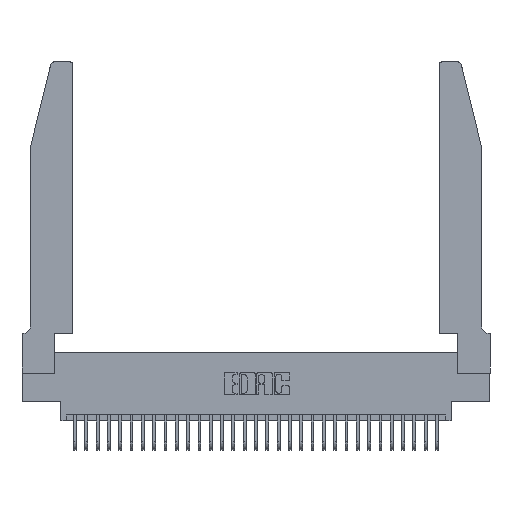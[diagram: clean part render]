
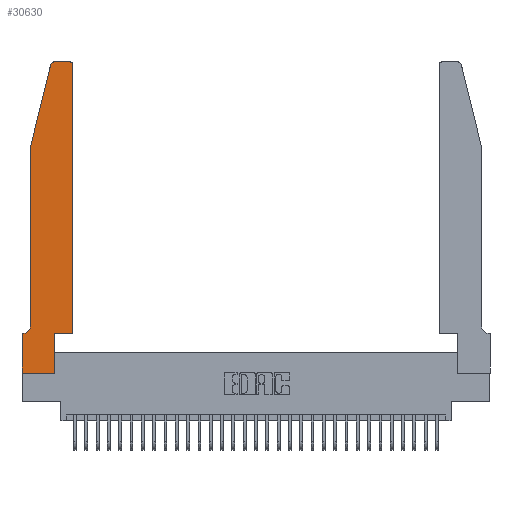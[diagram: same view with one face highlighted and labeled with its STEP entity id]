
A CAD part, top view. The second image highlights one B-rep face of the part: STEP entity #30630.
In plain terms, the highlighted planar face has unit normal (0, 0, 1).
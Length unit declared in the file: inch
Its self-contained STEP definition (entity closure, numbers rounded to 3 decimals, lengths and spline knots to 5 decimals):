
#262 = VECTOR ( 'NONE', #32092, 39.37008 ) ;
#339 = ORIENTED_EDGE ( 'NONE', *, *, #18833, .T. ) ;
#439 = CARTESIAN_POINT ( 'NONE',  ( 0.4205, 2.75, 0.37 ) ) ;
#1044 = EDGE_CURVE ( 'NONE', #23796, #20336, #15016, .T. ) ;
#1236 = EDGE_CURVE ( 'NONE', #20336, #14834, #1982, .T. ) ;
#1245 = VECTOR ( 'NONE', #25165, 39.37008 ) ;
#1545 = CARTESIAN_POINT ( 'NONE',  ( 0.25487, 2.72718, 0.37 ) ) ;
#1982 = CIRCLE ( 'NONE', #18334, 0.07 ) ;
#2623 = EDGE_LOOP ( 'NONE', ( #7126, #8928, #11662, #19348, #32763, #8503, #13892, #15949, #14632, #13035, #339, #10388 ) ) ;
#2801 = CARTESIAN_POINT ( 'NONE',  ( 0.0755, 2., 0.37 ) ) ;
#4645 = DIRECTION ( 'NONE',  ( 0., 1., 0. ) ) ;
#4680 = DIRECTION ( 'NONE',  ( 0., 0., -1. ) ) ;
#4824 = LINE ( 'NONE', #33565, #27201 ) ;
#4908 = DIRECTION ( 'NONE',  ( -1., 0., 0. ) ) ;
#6278 = VERTEX_POINT ( 'NONE', #18532 ) ;
#6332 = CARTESIAN_POINT ( 'NONE',  ( 0.284, 2.72, 0.37 ) ) ;
#6492 = DIRECTION ( 'NONE',  ( 1., 0., 0. ) ) ;
#7126 = ORIENTED_EDGE ( 'NONE', *, *, #12984, .T. ) ;
#7572 = VERTEX_POINT ( 'NONE', #22882 ) ;
#8291 = CARTESIAN_POINT ( 'NONE',  ( 0.0755, 2., 0.37 ) ) ;
#8503 = ORIENTED_EDGE ( 'NONE', *, *, #16036, .T. ) ;
#8522 = PLANE ( 'NONE',  #24957 ) ;
#8745 = DIRECTION ( 'NONE',  ( 1., 0., 0. ) ) ;
#8775 = CARTESIAN_POINT ( 'NONE',  ( 0.0055, 0.35, 0.37 ) ) ;
#8928 = ORIENTED_EDGE ( 'NONE', *, *, #31113, .T. ) ;
#9023 = CARTESIAN_POINT ( 'NONE',  ( 0.4505, 0.35, 0.37 ) ) ;
#9468 = DIRECTION ( 'NONE',  ( 0., -1., 0. ) ) ;
#9944 = VERTEX_POINT ( 'NONE', #31047 ) ;
#9985 = LINE ( 'NONE', #21358, #29141 ) ;
#10060 = EDGE_CURVE ( 'NONE', #6278, #31861, #24476, .T. ) ;
#10287 = DIRECTION ( 'NONE',  ( 1., 0., 0. ) ) ;
#10388 = ORIENTED_EDGE ( 'NONE', *, *, #11906, .T. ) ;
#11662 = ORIENTED_EDGE ( 'NONE', *, *, #32304, .T. ) ;
#11906 = EDGE_CURVE ( 'NONE', #7572, #33193, #21946, .T. ) ;
#12168 = EDGE_CURVE ( 'NONE', #9944, #29041, #4824, .T. ) ;
#12381 = FACE_OUTER_BOUND ( 'NONE', #2623, .T. ) ;
#12514 = AXIS2_PLACEMENT_3D ( 'NONE', #6332, #27166, #24223 ) ;
#12544 = CARTESIAN_POINT ( 'NONE',  ( 0., 0., 0.37 ) ) ;
#12796 = LINE ( 'NONE', #9023, #26636 ) ;
#12984 = EDGE_CURVE ( 'NONE', #33193, #17406, #9985, .T. ) ;
#13035 = ORIENTED_EDGE ( 'NONE', *, *, #16805, .T. ) ;
#13427 = VECTOR ( 'NONE', #18151, 39.37008 ) ;
#13646 = CARTESIAN_POINT ( 'NONE',  ( 0., 0., 0.37 ) ) ;
#13892 = ORIENTED_EDGE ( 'NONE', *, *, #10060, .T. ) ;
#14632 = ORIENTED_EDGE ( 'NONE', *, *, #12168, .T. ) ;
#14834 = VERTEX_POINT ( 'NONE', #8775 ) ;
#15016 = LINE ( 'NONE', #19865, #18705 ) ;
#15091 = VECTOR ( 'NONE', #10287, 39.37008 ) ;
#15474 = DIRECTION ( 'NONE',  ( 0., 1., 0. ) ) ;
#15493 = CARTESIAN_POINT ( 'NONE',  ( 0., 0., 0.37 ) ) ;
#15949 = ORIENTED_EDGE ( 'NONE', *, *, #26826, .T. ) ;
#16036 = EDGE_CURVE ( 'NONE', #14834, #6278, #31419, .T. ) ;
#16187 = CARTESIAN_POINT ( 'NONE',  ( 0., 0.35, 0.37 ) ) ;
#16805 = EDGE_CURVE ( 'NONE', #29041, #26132, #22052, .T. ) ;
#17406 = VERTEX_POINT ( 'NONE', #31102 ) ;
#17698 = CARTESIAN_POINT ( 'NONE',  ( 0.0755, 0.35, 0.37 ) ) ;
#18013 = CARTESIAN_POINT ( 'NONE',  ( 0.0755, 0.42, 0.37 ) ) ;
#18151 = DIRECTION ( 'NONE',  ( 1., 0., 0. ) ) ;
#18262 = DIRECTION ( 'NONE',  ( -1., 0., 0. ) ) ;
#18334 = AXIS2_PLACEMENT_3D ( 'NONE', #33453, #4680, #4908 ) ;
#18532 = CARTESIAN_POINT ( 'NONE',  ( 0., 0.35, 0.37 ) ) ;
#18705 = VECTOR ( 'NONE', #9468, 39.37008 ) ;
#18833 = EDGE_CURVE ( 'NONE', #26132, #7572, #12796, .T. ) ;
#19348 = ORIENTED_EDGE ( 'NONE', *, *, #1044, .T. ) ;
#19865 = CARTESIAN_POINT ( 'NONE',  ( 0.0755, 2., 0.37 ) ) ;
#20336 = VERTEX_POINT ( 'NONE', #18013 ) ;
#20381 = LINE ( 'NONE', #15493, #13427 ) ;
#21134 = DIRECTION ( 'NONE',  ( 0., 0., 1. ) ) ;
#21358 = CARTESIAN_POINT ( 'NONE',  ( 0.2605, 2.75, 0.37 ) ) ;
#21448 = DIRECTION ( 'NONE',  ( 0., 0., 1. ) ) ;
#21946 = CIRCLE ( 'NONE', #28947, 0.03 ) ;
#22052 = LINE ( 'NONE', #23327, #15091 ) ;
#22882 = CARTESIAN_POINT ( 'NONE',  ( 0.4505, 2.72, 0.37 ) ) ;
#23327 = CARTESIAN_POINT ( 'NONE',  ( 0.4505, 0.35, 0.37 ) ) ;
#23633 = CARTESIAN_POINT ( 'NONE',  ( 0.4205, 2.72, 0.37 ) ) ;
#23725 = VECTOR ( 'NONE', #18262, 39.37008 ) ;
#23796 = VERTEX_POINT ( 'NONE', #2801 ) ;
#24223 = DIRECTION ( 'NONE',  ( 1., 0., 0. ) ) ;
#24297 = DIRECTION ( 'NONE',  ( -1., 0., 0. ) ) ;
#24476 = LINE ( 'NONE', #13646, #1245 ) ;
#24957 = AXIS2_PLACEMENT_3D ( 'NONE', #16187, #21448, #6492 ) ;
#25165 = DIRECTION ( 'NONE',  ( 0., -1., 0. ) ) ;
#25671 = CARTESIAN_POINT ( 'NONE',  ( 0.4505, 0.35, 0.37 ) ) ;
#26029 = VERTEX_POINT ( 'NONE', #1545 ) ;
#26132 = VERTEX_POINT ( 'NONE', #25671 ) ;
#26636 = VECTOR ( 'NONE', #4645, 39.37008 ) ;
#26826 = EDGE_CURVE ( 'NONE', #31861, #9944, #20381, .T. ) ;
#27166 = DIRECTION ( 'NONE',  ( 0., 0., 1. ) ) ;
#27201 = VECTOR ( 'NONE', #15474, 39.37008 ) ;
#28356 = LINE ( 'NONE', #8291, #262 ) ;
#28947 = AXIS2_PLACEMENT_3D ( 'NONE', #23633, #21134, #8745 ) ;
#29041 = VERTEX_POINT ( 'NONE', #30691 ) ;
#29141 = VECTOR ( 'NONE', #24297, 39.37008 ) ;
#29439 = CIRCLE ( 'NONE', #12514, 0.03 ) ;
#30630 = ADVANCED_FACE ( 'NONE', ( #12381 ), #8522, .T. ) ;
#30691 = CARTESIAN_POINT ( 'NONE',  ( 0.2865, 0.35, 0.37 ) ) ;
#31047 = CARTESIAN_POINT ( 'NONE',  ( 0.2865, 0., 0.37 ) ) ;
#31102 = CARTESIAN_POINT ( 'NONE',  ( 0.284, 2.75, 0.37 ) ) ;
#31113 = EDGE_CURVE ( 'NONE', #17406, #26029, #29439, .T. ) ;
#31419 = LINE ( 'NONE', #17698, #23725 ) ;
#31861 = VERTEX_POINT ( 'NONE', #12544 ) ;
#32092 = DIRECTION ( 'NONE',  ( -0.239, -0.971, 0. ) ) ;
#32304 = EDGE_CURVE ( 'NONE', #26029, #23796, #28356, .T. ) ;
#32763 = ORIENTED_EDGE ( 'NONE', *, *, #1236, .T. ) ;
#33193 = VERTEX_POINT ( 'NONE', #439 ) ;
#33453 = CARTESIAN_POINT ( 'NONE',  ( 0.0055, 0.42, 0.37 ) ) ;
#33565 = CARTESIAN_POINT ( 'NONE',  ( 0.2865, 0.35, 0.37 ) ) ;
